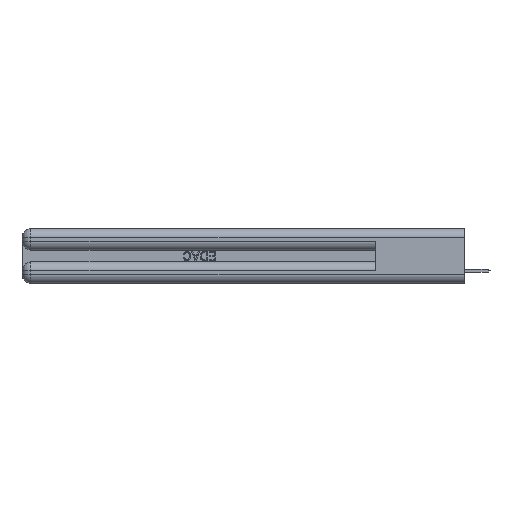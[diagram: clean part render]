
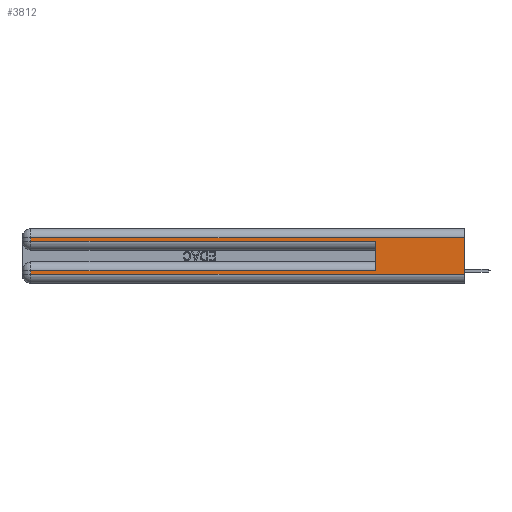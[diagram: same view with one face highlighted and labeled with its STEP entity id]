
A CAD part, left-side view. The second image highlights one B-rep face of the part: STEP entity #3812.
In plain terms, the highlighted planar face has unit normal (-1, 0, 0).
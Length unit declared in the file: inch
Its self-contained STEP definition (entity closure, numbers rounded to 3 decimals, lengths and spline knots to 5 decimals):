
#471 = EDGE_CURVE ( 'NONE', #22534, #16095, #15503, .T. ) ;
#1476 = CARTESIAN_POINT ( 'NONE',  ( 0., 0., 0.06 ) ) ;
#1503 = EDGE_CURVE ( 'NONE', #11282, #4107, #37744, .T. ) ;
#2983 = VECTOR ( 'NONE', #6088, 39.37008 ) ;
#3812 = ADVANCED_FACE ( 'NONE', ( #20132 ), #13459, .F. ) ;
#4107 = VERTEX_POINT ( 'NONE', #18374 ) ;
#4229 = ORIENTED_EDGE ( 'NONE', *, *, #19910, .T. ) ;
#4679 = ORIENTED_EDGE ( 'NONE', *, *, #28346, .T. ) ;
#6088 = DIRECTION ( 'NONE',  ( 0., 0., -1. ) ) ;
#6486 = DIRECTION ( 'NONE',  ( 0., -1., 0. ) ) ;
#6640 = EDGE_CURVE ( 'NONE', #16095, #13296, #7089, .T. ) ;
#7027 = CARTESIAN_POINT ( 'NONE',  ( 0., 0., 0.37 ) ) ;
#7089 = LINE ( 'NONE', #40544, #38543 ) ;
#7922 = ORIENTED_EDGE ( 'NONE', *, *, #1503, .F. ) ;
#8442 = CARTESIAN_POINT ( 'NONE',  ( 0., 0.6, 0.145 ) ) ;
#8813 = AXIS2_PLACEMENT_3D ( 'NONE', #7027, #38003, #37707 ) ;
#10061 = ORIENTED_EDGE ( 'NONE', *, *, #20260, .T. ) ;
#10460 = DIRECTION ( 'NONE',  ( 0., 0., -1. ) ) ;
#10822 = VECTOR ( 'NONE', #31437, 39.37008 ) ;
#11282 = VERTEX_POINT ( 'NONE', #33307 ) ;
#11343 = EDGE_CURVE ( 'NONE', #22534, #27791, #21333, .T. ) ;
#11380 = VECTOR ( 'NONE', #41657, 39.37008 ) ;
#12803 = ORIENTED_EDGE ( 'NONE', *, *, #471, .T. ) ;
#13252 = CARTESIAN_POINT ( 'NONE',  ( 0., 0., 0.085 ) ) ;
#13296 = VERTEX_POINT ( 'NONE', #35493 ) ;
#13459 = PLANE ( 'NONE',  #8813 ) ;
#14090 = CARTESIAN_POINT ( 'NONE',  ( 0., 0., 0.31 ) ) ;
#15027 = EDGE_CURVE ( 'NONE', #13296, #4107, #29247, .T. ) ;
#15503 = LINE ( 'NONE', #13252, #25239 ) ;
#15580 = DIRECTION ( 'NONE',  ( 0., 0., 1. ) ) ;
#16095 = VERTEX_POINT ( 'NONE', #32914 ) ;
#17556 = VECTOR ( 'NONE', #15580, 39.37008 ) ;
#18339 = ORIENTED_EDGE ( 'NONE', *, *, #6640, .T. ) ;
#18374 = CARTESIAN_POINT ( 'NONE',  ( 0., 0., 0.06 ) ) ;
#19910 = EDGE_CURVE ( 'NONE', #25711, #27791, #27935, .T. ) ;
#20132 = FACE_OUTER_BOUND ( 'NONE', #39916, .T. ) ;
#20260 = EDGE_CURVE ( 'NONE', #44365, #25711, #30619, .T. ) ;
#20874 = VECTOR ( 'NONE', #6486, 39.37008 ) ;
#21333 = LINE ( 'NONE', #8442, #17556 ) ;
#22534 = VERTEX_POINT ( 'NONE', #25441 ) ;
#23361 = CARTESIAN_POINT ( 'NONE',  ( 0., 0., 0.37 ) ) ;
#23382 = DIRECTION ( 'NONE',  ( 0., 1., 0. ) ) ;
#23962 = CARTESIAN_POINT ( 'NONE',  ( 0., 2.94, 0.37 ) ) ;
#24468 = ORIENTED_EDGE ( 'NONE', *, *, #15027, .T. ) ;
#25161 = VECTOR ( 'NONE', #10460, 39.37008 ) ;
#25239 = VECTOR ( 'NONE', #23382, 39.37008 ) ;
#25441 = CARTESIAN_POINT ( 'NONE',  ( 0., 0.6, 0.085 ) ) ;
#25451 = ORIENTED_EDGE ( 'NONE', *, *, #11343, .F. ) ;
#25711 = VERTEX_POINT ( 'NONE', #25938 ) ;
#25938 = CARTESIAN_POINT ( 'NONE',  ( 0., 2.94, 0.285 ) ) ;
#26360 = CARTESIAN_POINT ( 'NONE',  ( 0., 0., 0.285 ) ) ;
#27791 = VERTEX_POINT ( 'NONE', #37194 ) ;
#27935 = LINE ( 'NONE', #26360, #20874 ) ;
#28346 = EDGE_CURVE ( 'NONE', #11282, #44365, #31438, .T. ) ;
#29247 = LINE ( 'NONE', #1476, #10822 ) ;
#30619 = LINE ( 'NONE', #23962, #25161 ) ;
#31437 = DIRECTION ( 'NONE',  ( 0., -1., 0. ) ) ;
#31438 = LINE ( 'NONE', #14090, #11380 ) ;
#32914 = CARTESIAN_POINT ( 'NONE',  ( 0., 2.94, 0.085 ) ) ;
#33098 = DIRECTION ( 'NONE',  ( 0., 0., -1. ) ) ;
#33307 = CARTESIAN_POINT ( 'NONE',  ( 0., 0., 0.31 ) ) ;
#35493 = CARTESIAN_POINT ( 'NONE',  ( 0., 2.94, 0.06 ) ) ;
#37194 = CARTESIAN_POINT ( 'NONE',  ( 0., 0.6, 0.285 ) ) ;
#37707 = DIRECTION ( 'NONE',  ( 0., 0., -1. ) ) ;
#37744 = LINE ( 'NONE', #23361, #2983 ) ;
#38003 = DIRECTION ( 'NONE',  ( 1., 0., 0. ) ) ;
#38543 = VECTOR ( 'NONE', #33098, 39.37008 ) ;
#39694 = CARTESIAN_POINT ( 'NONE',  ( 0., 2.94, 0.31 ) ) ;
#39916 = EDGE_LOOP ( 'NONE', ( #7922, #4679, #10061, #4229, #25451, #12803, #18339, #24468 ) ) ;
#40544 = CARTESIAN_POINT ( 'NONE',  ( 0., 2.94, 0.37 ) ) ;
#41657 = DIRECTION ( 'NONE',  ( 0., 1., 0. ) ) ;
#44365 = VERTEX_POINT ( 'NONE', #39694 ) ;
